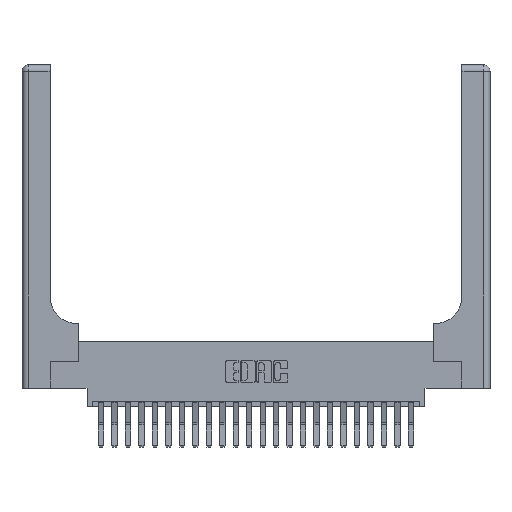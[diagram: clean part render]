
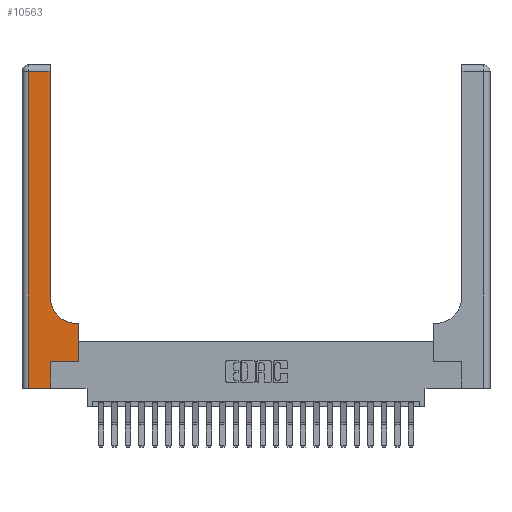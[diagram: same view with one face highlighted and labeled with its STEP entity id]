
A CAD part, top view. The second image highlights one B-rep face of the part: STEP entity #10563.
In plain terms, the highlighted planar face has unit normal (0, 0, 1).
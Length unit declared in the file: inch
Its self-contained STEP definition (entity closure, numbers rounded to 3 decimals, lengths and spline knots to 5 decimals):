
#114 = EDGE_CURVE ( 'NONE', #22551, #21454, #21330, .T. ) ;
#182 = FACE_OUTER_BOUND ( 'NONE', #22500, .T. ) ;
#384 = ORIENTED_EDGE ( 'NONE', *, *, #4557, .T. ) ;
#782 = EDGE_CURVE ( 'NONE', #18349, #14666, #13387, .T. ) ;
#1094 = LINE ( 'NONE', #8461, #23503 ) ;
#1438 = VECTOR ( 'NONE', #22223, 39.37008 ) ;
#1544 = VECTOR ( 'NONE', #18598, 39.37008 ) ;
#1976 = EDGE_CURVE ( 'NONE', #14666, #21423, #13699, .T. ) ;
#2096 = CARTESIAN_POINT ( 'NONE',  ( 0.06, 0., 0.37 ) ) ;
#3312 = VERTEX_POINT ( 'NONE', #10877 ) ;
#3437 = CARTESIAN_POINT ( 'NONE',  ( 0.265, 0., 0.37 ) ) ;
#3506 = EDGE_CURVE ( 'NONE', #17901, #9061, #8829, .T. ) ;
#3649 = VECTOR ( 'NONE', #11505, 39.37008 ) ;
#4557 = EDGE_CURVE ( 'NONE', #21454, #18349, #19383, .T. ) ;
#5360 = VECTOR ( 'NONE', #7860, 39.37008 ) ;
#5675 = CARTESIAN_POINT ( 'NONE',  ( 0.265, 0.25, 0.37 ) ) ;
#5704 = CARTESIAN_POINT ( 'NONE',  ( 0.26, 2.94, 0.37 ) ) ;
#5911 = CARTESIAN_POINT ( 'NONE',  ( 0.26, 3., 0.37 ) ) ;
#6326 = DIRECTION ( 'NONE',  ( 1., 0., 0. ) ) ;
#6650 = DIRECTION ( 'NONE',  ( -1., 0., 0. ) ) ;
#7322 = VECTOR ( 'NONE', #21448, 39.37008 ) ;
#7338 = LINE ( 'NONE', #14843, #1544 ) ;
#7860 = DIRECTION ( 'NONE',  ( 0., 1., 0. ) ) ;
#8126 = DIRECTION ( 'NONE',  ( 0., 0., -1. ) ) ;
#8211 = VERTEX_POINT ( 'NONE', #20455 ) ;
#8230 = DIRECTION ( 'NONE',  ( 0., 1., 0. ) ) ;
#8339 = CARTESIAN_POINT ( 'NONE',  ( 0.06, 2.94, 0.37 ) ) ;
#8461 = CARTESIAN_POINT ( 'NONE',  ( 0.26, 0.6, 0.37 ) ) ;
#8577 = ORIENTED_EDGE ( 'NONE', *, *, #15175, .T. ) ;
#8829 = CIRCLE ( 'NONE', #20809, 0.25 ) ;
#8979 = ORIENTED_EDGE ( 'NONE', *, *, #1976, .T. ) ;
#9061 = VERTEX_POINT ( 'NONE', #22580 ) ;
#9236 = ORIENTED_EDGE ( 'NONE', *, *, #782, .T. ) ;
#9245 = LINE ( 'NONE', #14816, #1438 ) ;
#9504 = ORIENTED_EDGE ( 'NONE', *, *, #16534, .T. ) ;
#10563 = ADVANCED_FACE ( 'NONE', ( #182 ), #13835, .F. ) ;
#10652 = ORIENTED_EDGE ( 'NONE', *, *, #114, .T. ) ;
#10877 = CARTESIAN_POINT ( 'NONE',  ( 0.528, 0.25, 0.37 ) ) ;
#11505 = DIRECTION ( 'NONE',  ( -1., 0., 0. ) ) ;
#11773 = VECTOR ( 'NONE', #8230, 39.37008 ) ;
#12034 = CARTESIAN_POINT ( 'NONE',  ( 0., 3., 0.37 ) ) ;
#12734 = ORIENTED_EDGE ( 'NONE', *, *, #15988, .T. ) ;
#13260 = CARTESIAN_POINT ( 'NONE',  ( 0.51, 0.6, 0.37 ) ) ;
#13387 = LINE ( 'NONE', #16899, #20611 ) ;
#13555 = LINE ( 'NONE', #5911, #5360 ) ;
#13688 = CARTESIAN_POINT ( 'NONE',  ( 0., 2.94, 0.37 ) ) ;
#13699 = LINE ( 'NONE', #19389, #11773 ) ;
#13835 = PLANE ( 'NONE',  #18799 ) ;
#14093 = DIRECTION ( 'NONE',  ( 0., 0., -1. ) ) ;
#14211 = EDGE_CURVE ( 'NONE', #21423, #3312, #7338, .T. ) ;
#14666 = VERTEX_POINT ( 'NONE', #3437 ) ;
#14816 = CARTESIAN_POINT ( 'NONE',  ( 0.528, 0.25, 0.37 ) ) ;
#14843 = CARTESIAN_POINT ( 'NONE',  ( 0.265, 0.25, 0.37 ) ) ;
#15175 = EDGE_CURVE ( 'NONE', #9061, #22551, #13555, .T. ) ;
#15669 = CARTESIAN_POINT ( 'NONE',  ( 0.51, 0.85, 0.37 ) ) ;
#15988 = EDGE_CURVE ( 'NONE', #3312, #8211, #9245, .T. ) ;
#16534 = EDGE_CURVE ( 'NONE', #8211, #17901, #1094, .T. ) ;
#16656 = ORIENTED_EDGE ( 'NONE', *, *, #3506, .T. ) ;
#16899 = CARTESIAN_POINT ( 'NONE',  ( 0., 0., 0.37 ) ) ;
#17901 = VERTEX_POINT ( 'NONE', #13260 ) ;
#18349 = VERTEX_POINT ( 'NONE', #2096 ) ;
#18598 = DIRECTION ( 'NONE',  ( 1., 0., 0. ) ) ;
#18799 = AXIS2_PLACEMENT_3D ( 'NONE', #12034, #8126, #22931 ) ;
#18823 = DIRECTION ( 'NONE',  ( 1., 0., 0. ) ) ;
#19383 = LINE ( 'NONE', #23273, #7322 ) ;
#19389 = CARTESIAN_POINT ( 'NONE',  ( 0.265, 0., 0.37 ) ) ;
#20455 = CARTESIAN_POINT ( 'NONE',  ( 0.528, 0.6, 0.37 ) ) ;
#20611 = VECTOR ( 'NONE', #18823, 39.37008 ) ;
#20809 = AXIS2_PLACEMENT_3D ( 'NONE', #15669, #14093, #6326 ) ;
#21330 = LINE ( 'NONE', #13688, #3649 ) ;
#21423 = VERTEX_POINT ( 'NONE', #5675 ) ;
#21448 = DIRECTION ( 'NONE',  ( 0., -1., 0. ) ) ;
#21454 = VERTEX_POINT ( 'NONE', #8339 ) ;
#22223 = DIRECTION ( 'NONE',  ( 0., 1., 0. ) ) ;
#22500 = EDGE_LOOP ( 'NONE', ( #8577, #10652, #384, #9236, #8979, #22755, #12734, #9504, #16656 ) ) ;
#22551 = VERTEX_POINT ( 'NONE', #5704 ) ;
#22580 = CARTESIAN_POINT ( 'NONE',  ( 0.26, 0.85, 0.37 ) ) ;
#22755 = ORIENTED_EDGE ( 'NONE', *, *, #14211, .T. ) ;
#22931 = DIRECTION ( 'NONE',  ( -1., 0., 0. ) ) ;
#23273 = CARTESIAN_POINT ( 'NONE',  ( 0.06, 3., 0.37 ) ) ;
#23503 = VECTOR ( 'NONE', #6650, 39.37008 ) ;
